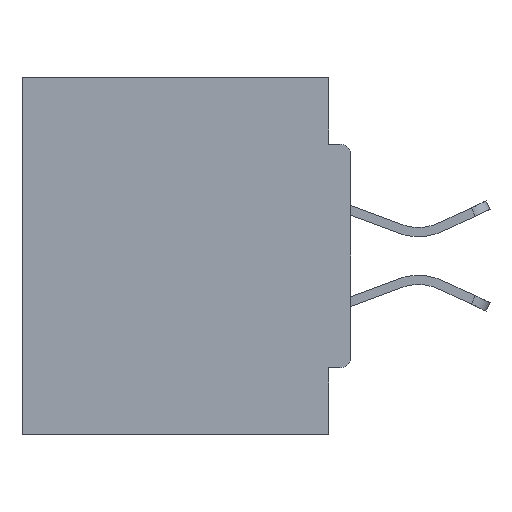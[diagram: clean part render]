
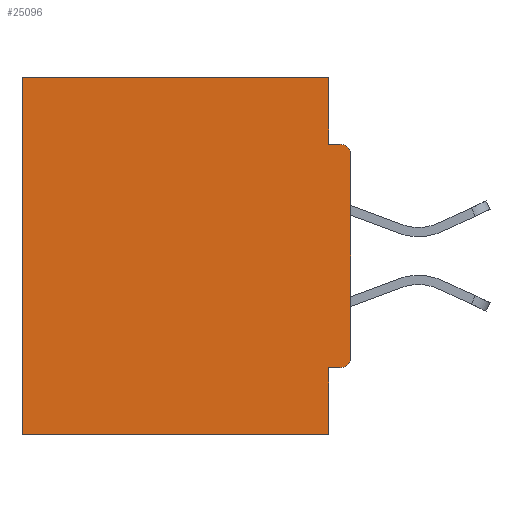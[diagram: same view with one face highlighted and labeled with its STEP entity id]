
A CAD part, left-side view. The second image highlights one B-rep face of the part: STEP entity #25096.
In plain terms, the highlighted planar face has unit normal (-1, 0, 0).
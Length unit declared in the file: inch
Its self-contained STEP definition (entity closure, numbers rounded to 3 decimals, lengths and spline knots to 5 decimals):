
#822 = DIRECTION ( 'NONE',  ( 0., -1., 0. ) ) ;
#1008 = DIRECTION ( 'NONE',  ( 0., 1., 0. ) ) ;
#1776 = DIRECTION ( 'NONE',  ( 0., 0., -1. ) ) ;
#1851 = DIRECTION ( 'NONE',  ( 0., 0., -1. ) ) ;
#2169 = VECTOR ( 'NONE', #3732, 39.37008 ) ;
#2260 = DIRECTION ( 'NONE',  ( 0., 1., 0. ) ) ;
#3500 = VERTEX_POINT ( 'NONE', #16984 ) ;
#3724 = VERTEX_POINT ( 'NONE', #3949 ) ;
#3732 = DIRECTION ( 'NONE',  ( 0., 0., -1. ) ) ;
#3805 = VERTEX_POINT ( 'NONE', #32795 ) ;
#3806 = DIRECTION ( 'NONE',  ( 0., 0., -1. ) ) ;
#3949 = CARTESIAN_POINT ( 'NONE',  ( 0.298, 0.031, -0.4065 ) ) ;
#4095 = EDGE_CURVE ( 'NONE', #34024, #33406, #18920, .T. ) ;
#5078 = ORIENTED_EDGE ( 'NONE', *, *, #7928, .T. ) ;
#5231 = DIRECTION ( 'NONE',  ( 0., 0., -1. ) ) ;
#5269 = VECTOR ( 'NONE', #1008, 39.37008 ) ;
#5359 = AXIS2_PLACEMENT_3D ( 'NONE', #11043, #31381, #5566 ) ;
#5566 = DIRECTION ( 'NONE',  ( 0., 0., -1. ) ) ;
#5634 = ORIENTED_EDGE ( 'NONE', *, *, #26164, .F. ) ;
#5675 = LINE ( 'NONE', #29994, #35695 ) ;
#6311 = AXIS2_PLACEMENT_3D ( 'NONE', #34089, #19998, #5231 ) ;
#7928 = EDGE_CURVE ( 'NONE', #3500, #9074, #33094, .T. ) ;
#8446 = VECTOR ( 'NONE', #2260, 39.37008 ) ;
#8858 = LINE ( 'NONE', #15806, #32915 ) ;
#9074 = VERTEX_POINT ( 'NONE', #30159 ) ;
#9600 = ORIENTED_EDGE ( 'NONE', *, *, #16754, .F. ) ;
#9722 = EDGE_CURVE ( 'NONE', #3724, #12731, #18115, .T. ) ;
#9866 = CARTESIAN_POINT ( 'NONE',  ( 0.298, 0.031, -0.5 ) ) ;
#11043 = CARTESIAN_POINT ( 'NONE',  ( 0.298, 0.015, -0.1085 ) ) ;
#11641 = EDGE_CURVE ( 'NONE', #12731, #33865, #31205, .T. ) ;
#12063 = VECTOR ( 'NONE', #37108, 39.37008 ) ;
#12292 = ORIENTED_EDGE ( 'NONE', *, *, #4095, .T. ) ;
#12684 = VERTEX_POINT ( 'NONE', #18244 ) ;
#12731 = VERTEX_POINT ( 'NONE', #9866 ) ;
#13045 = ORIENTED_EDGE ( 'NONE', *, *, #29777, .F. ) ;
#13394 = CARTESIAN_POINT ( 'NONE',  ( 0.298, 0.46, 0. ) ) ;
#13821 = VECTOR ( 'NONE', #27305, 39.37008 ) ;
#13842 = PLANE ( 'NONE',  #30076 ) ;
#13887 = LINE ( 'NONE', #25641, #12063 ) ;
#13893 = VECTOR ( 'NONE', #1776, 39.37008 ) ;
#14603 = CARTESIAN_POINT ( 'NONE',  ( 0.298, 0.031, -0.5 ) ) ;
#15190 = LINE ( 'NONE', #30398, #13821 ) ;
#15716 = CARTESIAN_POINT ( 'NONE',  ( 0.298, 0., -0.5 ) ) ;
#15806 = CARTESIAN_POINT ( 'NONE',  ( 0.298, 0., 0. ) ) ;
#16754 = EDGE_CURVE ( 'NONE', #3500, #3724, #13887, .T. ) ;
#16984 = CARTESIAN_POINT ( 'NONE',  ( 0.298, 0.015, -0.4065 ) ) ;
#17881 = ORIENTED_EDGE ( 'NONE', *, *, #33915, .F. ) ;
#18115 = LINE ( 'NONE', #14603, #2169 ) ;
#18244 = CARTESIAN_POINT ( 'NONE',  ( 0.298, 0.031, -0.0935 ) ) ;
#18703 = CARTESIAN_POINT ( 'NONE',  ( 0.298, 0.46, -0.5 ) ) ;
#18920 = LINE ( 'NONE', #22408, #8446 ) ;
#19789 = CARTESIAN_POINT ( 'NONE',  ( 0.298, 0.015, -0.0935 ) ) ;
#19998 = DIRECTION ( 'NONE',  ( -1., 0., 0. ) ) ;
#22365 = CARTESIAN_POINT ( 'NONE',  ( 0.298, 0., 0. ) ) ;
#22408 = CARTESIAN_POINT ( 'NONE',  ( 0.298, 0., 0. ) ) ;
#23137 = ORIENTED_EDGE ( 'NONE', *, *, #31359, .T. ) ;
#24962 = CARTESIAN_POINT ( 'NONE',  ( 0.298, 0.031, -0.5 ) ) ;
#25096 = ADVANCED_FACE ( 'NONE', ( #29793 ), #13842, .F. ) ;
#25259 = LINE ( 'NONE', #24962, #13893 ) ;
#25641 = CARTESIAN_POINT ( 'NONE',  ( 0.298, 0., -0.4065 ) ) ;
#26164 = EDGE_CURVE ( 'NONE', #3805, #9074, #8858, .T. ) ;
#27110 = EDGE_LOOP ( 'NONE', ( #30638, #17881, #13045, #12292, #23137, #30801, #29233, #9600, #5078, #5634 ) ) ;
#27305 = DIRECTION ( 'NONE',  ( 0., 0., -1. ) ) ;
#29233 = ORIENTED_EDGE ( 'NONE', *, *, #9722, .F. ) ;
#29777 = EDGE_CURVE ( 'NONE', #34024, #12684, #25259, .T. ) ;
#29793 = FACE_OUTER_BOUND ( 'NONE', #27110, .T. ) ;
#29968 = EDGE_CURVE ( 'NONE', #3805, #36009, #36131, .T. ) ;
#29994 = CARTESIAN_POINT ( 'NONE',  ( 0.298, 0., -0.0935 ) ) ;
#30076 = AXIS2_PLACEMENT_3D ( 'NONE', #22365, #34037, #1851 ) ;
#30159 = CARTESIAN_POINT ( 'NONE',  ( 0.298, 0., -0.3915 ) ) ;
#30398 = CARTESIAN_POINT ( 'NONE',  ( 0.298, 0.46, 0. ) ) ;
#30638 = ORIENTED_EDGE ( 'NONE', *, *, #29968, .T. ) ;
#30801 = ORIENTED_EDGE ( 'NONE', *, *, #11641, .F. ) ;
#31205 = LINE ( 'NONE', #15716, #5269 ) ;
#31359 = EDGE_CURVE ( 'NONE', #33406, #33865, #15190, .T. ) ;
#31381 = DIRECTION ( 'NONE',  ( -1., 0., 0. ) ) ;
#32795 = CARTESIAN_POINT ( 'NONE',  ( 0.298, 0., -0.1085 ) ) ;
#32915 = VECTOR ( 'NONE', #3806, 39.37008 ) ;
#33094 = CIRCLE ( 'NONE', #6311, 0.015 ) ;
#33406 = VERTEX_POINT ( 'NONE', #13394 ) ;
#33865 = VERTEX_POINT ( 'NONE', #18703 ) ;
#33915 = EDGE_CURVE ( 'NONE', #12684, #36009, #5675, .T. ) ;
#33917 = CARTESIAN_POINT ( 'NONE',  ( 0.298, 0.031, 0. ) ) ;
#34024 = VERTEX_POINT ( 'NONE', #33917 ) ;
#34037 = DIRECTION ( 'NONE',  ( 1., 0., 0. ) ) ;
#34089 = CARTESIAN_POINT ( 'NONE',  ( 0.298, 0.015, -0.3915 ) ) ;
#35695 = VECTOR ( 'NONE', #822, 39.37008 ) ;
#36009 = VERTEX_POINT ( 'NONE', #19789 ) ;
#36131 = CIRCLE ( 'NONE', #5359, 0.015 ) ;
#37108 = DIRECTION ( 'NONE',  ( 0., 1., 0. ) ) ;
